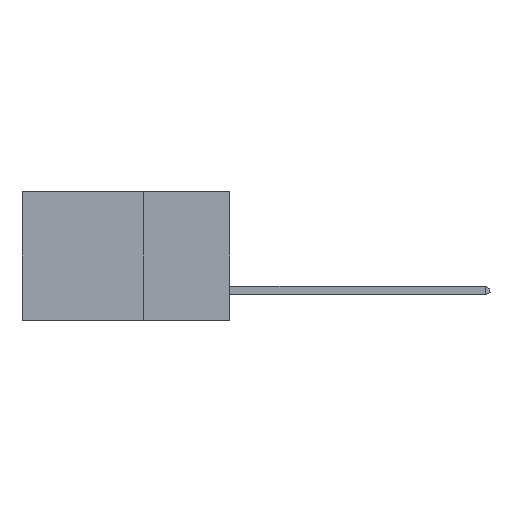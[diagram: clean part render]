
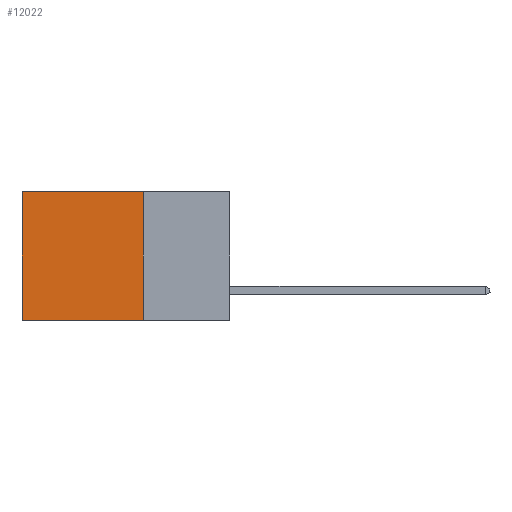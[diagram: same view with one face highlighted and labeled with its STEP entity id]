
A CAD part, left-side view. The second image highlights one B-rep face of the part: STEP entity #12022.
In plain terms, the highlighted planar face has unit normal (-1, 0, 0).
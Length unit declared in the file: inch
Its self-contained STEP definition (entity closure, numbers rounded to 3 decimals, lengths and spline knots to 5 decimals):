
#1449 = LINE ( 'NONE', #12861, #14954 ) ;
#2818 = EDGE_LOOP ( 'NONE', ( #20560, #15133, #8222, #9554 ) ) ;
#5227 = VERTEX_POINT ( 'NONE', #8699 ) ;
#8162 = DIRECTION ( 'NONE',  ( 1., 0., 0. ) ) ;
#8222 = ORIENTED_EDGE ( 'NONE', *, *, #10370, .F. ) ;
#8699 = CARTESIAN_POINT ( 'NONE',  ( 0.298, 0.25, -0.37 ) ) ;
#8760 = CARTESIAN_POINT ( 'NONE',  ( 0.298, 0.6, 0. ) ) ;
#9090 = DIRECTION ( 'NONE',  ( 0., 1., 0. ) ) ;
#9554 = ORIENTED_EDGE ( 'NONE', *, *, #15253, .T. ) ;
#9968 = CARTESIAN_POINT ( 'NONE',  ( 0.298, 0.25, -0.37 ) ) ;
#10370 = EDGE_CURVE ( 'NONE', #15223, #5227, #18504, .T. ) ;
#12022 = ADVANCED_FACE ( 'NONE', ( #18723 ), #12104, .F. ) ;
#12104 = PLANE ( 'NONE',  #14723 ) ;
#12602 = CARTESIAN_POINT ( 'NONE',  ( 0.298, 0.25, 0. ) ) ;
#12861 = CARTESIAN_POINT ( 'NONE',  ( 0.298, 0.25, 0. ) ) ;
#13407 = VECTOR ( 'NONE', #23312, 39.37008 ) ;
#14723 = AXIS2_PLACEMENT_3D ( 'NONE', #15987, #8162, #16074 ) ;
#14764 = CARTESIAN_POINT ( 'NONE',  ( 0.298, 0.6, 0. ) ) ;
#14954 = VECTOR ( 'NONE', #9090, 39.37008 ) ;
#15133 = ORIENTED_EDGE ( 'NONE', *, *, #20830, .F. ) ;
#15223 = VERTEX_POINT ( 'NONE', #12602 ) ;
#15243 = VERTEX_POINT ( 'NONE', #8760 ) ;
#15253 = EDGE_CURVE ( 'NONE', #15223, #15243, #1449, .T. ) ;
#15929 = LINE ( 'NONE', #14764, #23118 ) ;
#15987 = CARTESIAN_POINT ( 'NONE',  ( 0.298, 0.25, 0. ) ) ;
#16074 = DIRECTION ( 'NONE',  ( 0., 0., -1. ) ) ;
#17353 = VERTEX_POINT ( 'NONE', #24655 ) ;
#17534 = CARTESIAN_POINT ( 'NONE',  ( 0.298, 0.25, 0. ) ) ;
#17620 = DIRECTION ( 'NONE',  ( 0., 1., 0. ) ) ;
#17628 = EDGE_CURVE ( 'NONE', #15243, #17353, #15929, .T. ) ;
#18504 = LINE ( 'NONE', #17534, #13407 ) ;
#18610 = DIRECTION ( 'NONE',  ( 0., 0., -1. ) ) ;
#18723 = FACE_OUTER_BOUND ( 'NONE', #2818, .T. ) ;
#20560 = ORIENTED_EDGE ( 'NONE', *, *, #17628, .T. ) ;
#20830 = EDGE_CURVE ( 'NONE', #5227, #17353, #24113, .T. ) ;
#23118 = VECTOR ( 'NONE', #18610, 39.37008 ) ;
#23312 = DIRECTION ( 'NONE',  ( 0., 0., -1. ) ) ;
#23515 = VECTOR ( 'NONE', #17620, 39.37008 ) ;
#24113 = LINE ( 'NONE', #9968, #23515 ) ;
#24655 = CARTESIAN_POINT ( 'NONE',  ( 0.298, 0.6, -0.37 ) ) ;
